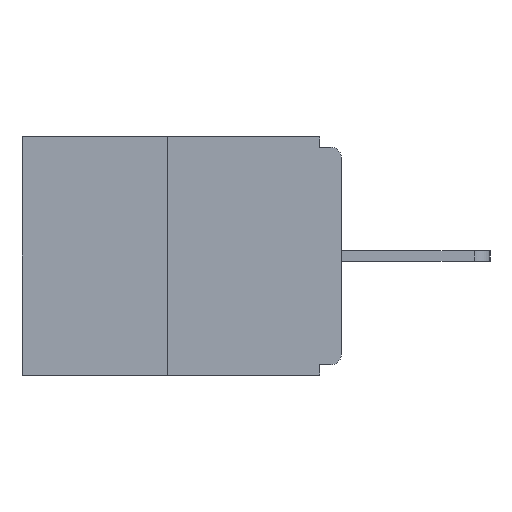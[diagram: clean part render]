
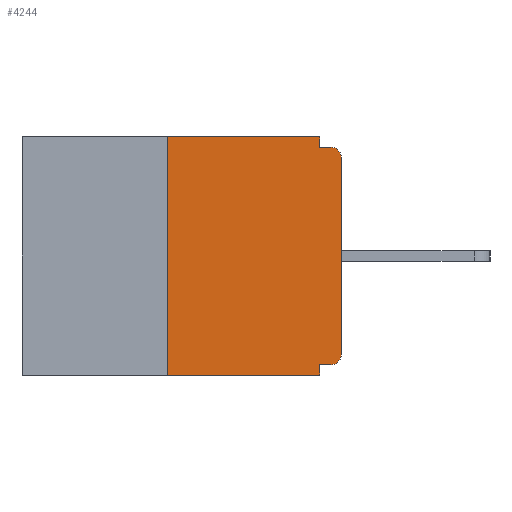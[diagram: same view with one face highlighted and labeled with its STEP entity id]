
A CAD part, left-side view. The second image highlights one B-rep face of the part: STEP entity #4244.
In plain terms, the highlighted planar face has unit normal (-1, 0, 0).
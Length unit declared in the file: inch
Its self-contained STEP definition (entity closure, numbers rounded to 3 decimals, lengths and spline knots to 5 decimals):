
#182 = CARTESIAN_POINT ( 'NONE',  ( 0., 0.031, 0. ) ) ;
#578 = FACE_OUTER_BOUND ( 'NONE', #8143, .T. ) ;
#700 = CARTESIAN_POINT ( 'NONE',  ( 0., 0.46, 0. ) ) ;
#764 = LINE ( 'NONE', #13339, #7172 ) ;
#1317 = CARTESIAN_POINT ( 'NONE',  ( 0., 0., -0.015 ) ) ;
#1413 = VERTEX_POINT ( 'NONE', #9981 ) ;
#1874 = CARTESIAN_POINT ( 'NONE',  ( 0., 0., -0.03 ) ) ;
#2002 = CARTESIAN_POINT ( 'NONE',  ( 0., 0.015, -0.328 ) ) ;
#2176 = AXIS2_PLACEMENT_3D ( 'NONE', #14479, #7108, #15677 ) ;
#2251 = PLANE ( 'NONE',  #10026 ) ;
#2398 = DIRECTION ( 'NONE',  ( 0., 0., -1. ) ) ;
#2475 = LINE ( 'NONE', #5570, #10995 ) ;
#2717 = ORIENTED_EDGE ( 'NONE', *, *, #6019, .T. ) ;
#2783 = EDGE_CURVE ( 'NONE', #4242, #15296, #2475, .T. ) ;
#2821 = CARTESIAN_POINT ( 'NONE',  ( 0., 0., -0.328 ) ) ;
#2972 = CARTESIAN_POINT ( 'NONE',  ( 0., 0.031, -0.328 ) ) ;
#3013 = LINE ( 'NONE', #700, #5608 ) ;
#3015 = CARTESIAN_POINT ( 'NONE',  ( 0., 0.25, 0. ) ) ;
#3104 = VERTEX_POINT ( 'NONE', #3681 ) ;
#3168 = CIRCLE ( 'NONE', #15479, 0.015 ) ;
#3234 = DIRECTION ( 'NONE',  ( -1., 0., 0. ) ) ;
#3681 = CARTESIAN_POINT ( 'NONE',  ( 0., 0.031, -0.015 ) ) ;
#4234 = LINE ( 'NONE', #1317, #13776 ) ;
#4242 = VERTEX_POINT ( 'NONE', #13225 ) ;
#4244 = ADVANCED_FACE ( 'NONE', ( #578 ), #2251, .F. ) ;
#4393 = EDGE_CURVE ( 'NONE', #9645, #8970, #12058, .T. ) ;
#4482 = DIRECTION ( 'NONE',  ( 0., 0., -1. ) ) ;
#4489 = CARTESIAN_POINT ( 'NONE',  ( 0., 0.46, -0.343 ) ) ;
#4559 = EDGE_CURVE ( 'NONE', #15296, #1413, #3013, .T. ) ;
#4872 = VECTOR ( 'NONE', #4482, 39.37008 ) ;
#4907 = EDGE_CURVE ( 'NONE', #7893, #13183, #764, .T. ) ;
#4919 = ORIENTED_EDGE ( 'NONE', *, *, #4393, .F. ) ;
#5013 = VECTOR ( 'NONE', #12342, 39.37008 ) ;
#5281 = LINE ( 'NONE', #5759, #4872 ) ;
#5511 = DIRECTION ( 'NONE',  ( 0., -1., 0. ) ) ;
#5570 = CARTESIAN_POINT ( 'NONE',  ( 0., 0.25, 0. ) ) ;
#5608 = VECTOR ( 'NONE', #5511, 39.37008 ) ;
#5759 = CARTESIAN_POINT ( 'NONE',  ( 0., 0.031, -0.343 ) ) ;
#6019 = EDGE_CURVE ( 'NONE', #13183, #15222, #3168, .T. ) ;
#7102 = ORIENTED_EDGE ( 'NONE', *, *, #4559, .F. ) ;
#7108 = DIRECTION ( 'NONE',  ( -1., 0., 0. ) ) ;
#7172 = VECTOR ( 'NONE', #7697, 39.37008 ) ;
#7475 = LINE ( 'NONE', #182, #8286 ) ;
#7488 = ORIENTED_EDGE ( 'NONE', *, *, #2783, .F. ) ;
#7697 = DIRECTION ( 'NONE',  ( 0., 0., 1. ) ) ;
#7893 = VERTEX_POINT ( 'NONE', #11795 ) ;
#7898 = CARTESIAN_POINT ( 'NONE',  ( 0., 0.015, -0.015 ) ) ;
#8143 = EDGE_LOOP ( 'NONE', ( #7102, #7488, #10855, #14418, #4919, #11590, #11968, #2717, #9920, #13106 ) ) ;
#8227 = EDGE_CURVE ( 'NONE', #1413, #3104, #7475, .T. ) ;
#8286 = VECTOR ( 'NONE', #9183, 39.37008 ) ;
#8820 = VERTEX_POINT ( 'NONE', #15140 ) ;
#8970 = VERTEX_POINT ( 'NONE', #2972 ) ;
#8983 = DIRECTION ( 'NONE',  ( 0., -1., 0. ) ) ;
#9009 = LINE ( 'NONE', #4489, #11496 ) ;
#9090 = EDGE_CURVE ( 'NONE', #8970, #8820, #5281, .T. ) ;
#9154 = CIRCLE ( 'NONE', #2176, 0.015 ) ;
#9183 = DIRECTION ( 'NONE',  ( 0., 0., -1. ) ) ;
#9624 = DIRECTION ( 'NONE',  ( 0., -1., 0. ) ) ;
#9645 = VERTEX_POINT ( 'NONE', #2002 ) ;
#9665 = DIRECTION ( 'NONE',  ( 0., 0., 1. ) ) ;
#9920 = ORIENTED_EDGE ( 'NONE', *, *, #15111, .F. ) ;
#9981 = CARTESIAN_POINT ( 'NONE',  ( 0., 0.031, 0. ) ) ;
#10026 = AXIS2_PLACEMENT_3D ( 'NONE', #13884, #14371, #2398 ) ;
#10270 = EDGE_CURVE ( 'NONE', #9645, #7893, #9154, .T. ) ;
#10815 = CARTESIAN_POINT ( 'NONE',  ( 0., 0.015, -0.03 ) ) ;
#10855 = ORIENTED_EDGE ( 'NONE', *, *, #14781, .T. ) ;
#10995 = VECTOR ( 'NONE', #9665, 39.37008 ) ;
#11496 = VECTOR ( 'NONE', #9624, 39.37008 ) ;
#11590 = ORIENTED_EDGE ( 'NONE', *, *, #10270, .T. ) ;
#11795 = CARTESIAN_POINT ( 'NONE',  ( 0., 0., -0.313 ) ) ;
#11968 = ORIENTED_EDGE ( 'NONE', *, *, #4907, .T. ) ;
#12011 = DIRECTION ( 'NONE',  ( 0., 0., -1. ) ) ;
#12058 = LINE ( 'NONE', #2821, #5013 ) ;
#12342 = DIRECTION ( 'NONE',  ( 0., 1., 0. ) ) ;
#13106 = ORIENTED_EDGE ( 'NONE', *, *, #8227, .F. ) ;
#13183 = VERTEX_POINT ( 'NONE', #1874 ) ;
#13225 = CARTESIAN_POINT ( 'NONE',  ( 0., 0.25, -0.343 ) ) ;
#13339 = CARTESIAN_POINT ( 'NONE',  ( 0., 0., 0. ) ) ;
#13776 = VECTOR ( 'NONE', #8983, 39.37008 ) ;
#13884 = CARTESIAN_POINT ( 'NONE',  ( 0., 0.46, 0. ) ) ;
#14371 = DIRECTION ( 'NONE',  ( 1., 0., 0. ) ) ;
#14418 = ORIENTED_EDGE ( 'NONE', *, *, #9090, .F. ) ;
#14479 = CARTESIAN_POINT ( 'NONE',  ( 0., 0.015, -0.313 ) ) ;
#14781 = EDGE_CURVE ( 'NONE', #4242, #8820, #9009, .T. ) ;
#15111 = EDGE_CURVE ( 'NONE', #3104, #15222, #4234, .T. ) ;
#15140 = CARTESIAN_POINT ( 'NONE',  ( 0., 0.031, -0.343 ) ) ;
#15222 = VERTEX_POINT ( 'NONE', #7898 ) ;
#15296 = VERTEX_POINT ( 'NONE', #3015 ) ;
#15479 = AXIS2_PLACEMENT_3D ( 'NONE', #10815, #3234, #12011 ) ;
#15677 = DIRECTION ( 'NONE',  ( 0., 0., -1. ) ) ;
